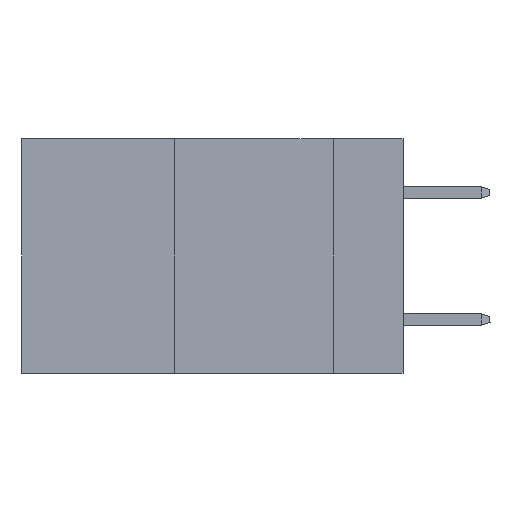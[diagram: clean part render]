
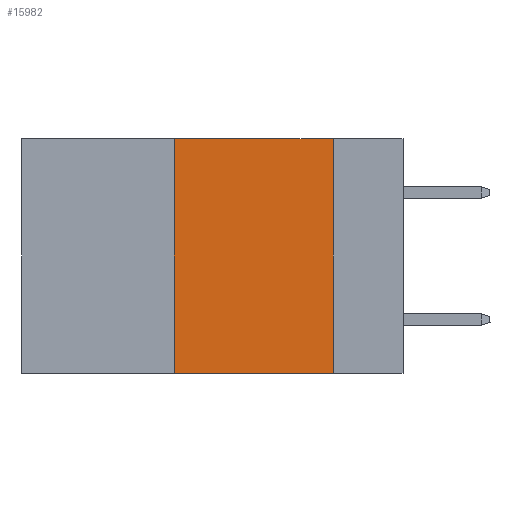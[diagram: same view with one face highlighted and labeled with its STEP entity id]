
A CAD part, left-side view. The second image highlights one B-rep face of the part: STEP entity #15982.
In plain terms, the highlighted planar face has unit normal (-1, 0, 0).
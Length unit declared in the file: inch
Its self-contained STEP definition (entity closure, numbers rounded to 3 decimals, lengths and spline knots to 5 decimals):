
#995 = VERTEX_POINT ( 'NONE', #25381 ) ;
#4799 = VERTEX_POINT ( 'NONE', #6582 ) ;
#6582 = CARTESIAN_POINT ( 'NONE',  ( 0., 0.11, 0. ) ) ;
#9203 = EDGE_CURVE ( 'NONE', #23724, #4799, #9673, .T. ) ;
#9346 = CARTESIAN_POINT ( 'NONE',  ( 0., 0.6, 0. ) ) ;
#9664 = FACE_OUTER_BOUND ( 'NONE', #29085, .T. ) ;
#9673 = LINE ( 'NONE', #21642, #16980 ) ;
#11315 = LINE ( 'NONE', #22837, #11613 ) ;
#11613 = VECTOR ( 'NONE', #16482, 39.37008 ) ;
#12081 = PLANE ( 'NONE',  #13446 ) ;
#12183 = LINE ( 'NONE', #17362, #16397 ) ;
#12927 = CARTESIAN_POINT ( 'NONE',  ( 0., 0.11, -0.37 ) ) ;
#13446 = AXIS2_PLACEMENT_3D ( 'NONE', #9346, #26308, #21951 ) ;
#13574 = VERTEX_POINT ( 'NONE', #12927 ) ;
#13738 = ORIENTED_EDGE ( 'NONE', *, *, #19734, .T. ) ;
#15982 = ADVANCED_FACE ( 'NONE', ( #9664 ), #12081, .F. ) ;
#16397 = VECTOR ( 'NONE', #19938, 39.37008 ) ;
#16482 = DIRECTION ( 'NONE',  ( 0., 0., 1. ) ) ;
#16980 = VECTOR ( 'NONE', #26631, 39.37008 ) ;
#17362 = CARTESIAN_POINT ( 'NONE',  ( 0., 0.11, 0. ) ) ;
#17397 = ORIENTED_EDGE ( 'NONE', *, *, #30972, .F. ) ;
#17796 = CARTESIAN_POINT ( 'NONE',  ( 0., 0.36, 0. ) ) ;
#18780 = VECTOR ( 'NONE', #21209, 39.37008 ) ;
#19734 = EDGE_CURVE ( 'NONE', #995, #13574, #23628, .T. ) ;
#19938 = DIRECTION ( 'NONE',  ( 0., 0., -1. ) ) ;
#21209 = DIRECTION ( 'NONE',  ( 0., -1., 0. ) ) ;
#21596 = EDGE_CURVE ( 'NONE', #995, #23724, #11315, .T. ) ;
#21642 = CARTESIAN_POINT ( 'NONE',  ( 0., 0.6, 0. ) ) ;
#21687 = ORIENTED_EDGE ( 'NONE', *, *, #9203, .F. ) ;
#21951 = DIRECTION ( 'NONE',  ( 0., 0., -1. ) ) ;
#22837 = CARTESIAN_POINT ( 'NONE',  ( 0., 0.36, 0. ) ) ;
#23628 = LINE ( 'NONE', #28631, #18780 ) ;
#23724 = VERTEX_POINT ( 'NONE', #17796 ) ;
#25381 = CARTESIAN_POINT ( 'NONE',  ( 0., 0.36, -0.37 ) ) ;
#26308 = DIRECTION ( 'NONE',  ( 1., 0., 0. ) ) ;
#26631 = DIRECTION ( 'NONE',  ( 0., -1., 0. ) ) ;
#28631 = CARTESIAN_POINT ( 'NONE',  ( 0., 0.6, -0.37 ) ) ;
#29085 = EDGE_LOOP ( 'NONE', ( #17397, #21687, #29395, #13738 ) ) ;
#29395 = ORIENTED_EDGE ( 'NONE', *, *, #21596, .F. ) ;
#30972 = EDGE_CURVE ( 'NONE', #4799, #13574, #12183, .T. ) ;
